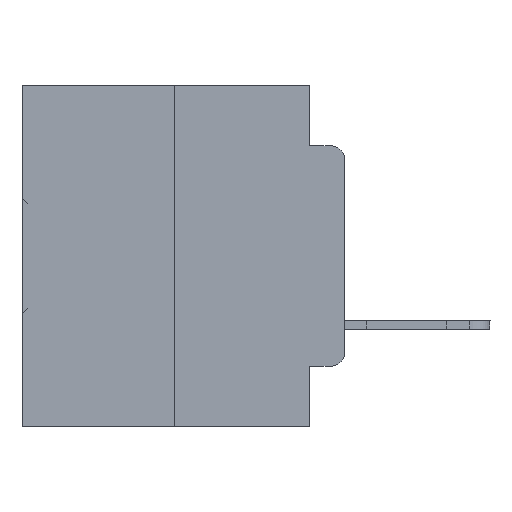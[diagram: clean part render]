
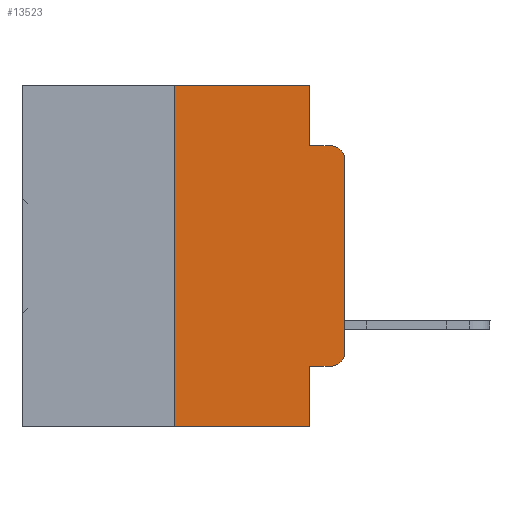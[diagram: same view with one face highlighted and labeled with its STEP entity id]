
A CAD part, left-side view. The second image highlights one B-rep face of the part: STEP entity #13523.
In plain terms, the highlighted planar face has unit normal (-1, 0, 0).
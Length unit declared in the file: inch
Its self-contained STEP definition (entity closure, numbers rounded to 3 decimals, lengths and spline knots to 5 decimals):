
#592 = EDGE_LOOP ( 'NONE', ( #31314, #16976, #10847, #1196, #27279, #27084, #24751, #25529, #22834, #14089 ) ) ;
#767 = CIRCLE ( 'NONE', #9210, 0.02 ) ;
#1196 = ORIENTED_EDGE ( 'NONE', *, *, #12137, .F. ) ;
#1541 = EDGE_CURVE ( 'NONE', #3699, #8849, #767, .T. ) ;
#2777 = DIRECTION ( 'NONE',  ( -1., 0., 0. ) ) ;
#3699 = VERTEX_POINT ( 'NONE', #29137 ) ;
#4284 = VECTOR ( 'NONE', #35732, 39.37008 ) ;
#4747 = CARTESIAN_POINT ( 'NONE',  ( 0., 0.051, -0.0885 ) ) ;
#5040 = DIRECTION ( 'NONE',  ( 0., 0., -1. ) ) ;
#5095 = VERTEX_POINT ( 'NONE', #4747 ) ;
#5227 = CARTESIAN_POINT ( 'NONE',  ( 0., 0.02, -0.3915 ) ) ;
#5934 = CARTESIAN_POINT ( 'NONE',  ( 0., 0.02, -0.1085 ) ) ;
#6182 = DIRECTION ( 'NONE',  ( 0., 0., 1. ) ) ;
#6283 = LINE ( 'NONE', #27998, #31683 ) ;
#6561 = CARTESIAN_POINT ( 'NONE',  ( 0., 0., -0.3915 ) ) ;
#7184 = CARTESIAN_POINT ( 'NONE',  ( 0., 0.25, -0.5 ) ) ;
#7583 = VERTEX_POINT ( 'NONE', #31201 ) ;
#8425 = LINE ( 'NONE', #22892, #10570 ) ;
#8849 = VERTEX_POINT ( 'NONE', #6561 ) ;
#9210 = AXIS2_PLACEMENT_3D ( 'NONE', #5227, #2777, #22008 ) ;
#10047 = VECTOR ( 'NONE', #14059, 39.37008 ) ;
#10087 = DIRECTION ( 'NONE',  ( 0., 0., 1. ) ) ;
#10299 = CARTESIAN_POINT ( 'NONE',  ( 0., 0.051, 0. ) ) ;
#10502 = VERTEX_POINT ( 'NONE', #25774 ) ;
#10570 = VECTOR ( 'NONE', #33578, 39.37008 ) ;
#10847 = ORIENTED_EDGE ( 'NONE', *, *, #14008, .F. ) ;
#11487 = VECTOR ( 'NONE', #10087, 39.37008 ) ;
#11555 = LINE ( 'NONE', #27419, #4284 ) ;
#11594 = EDGE_CURVE ( 'NONE', #13552, #33379, #26052, .T. ) ;
#12137 = EDGE_CURVE ( 'NONE', #33379, #5095, #21808, .T. ) ;
#12580 = CARTESIAN_POINT ( 'NONE',  ( 0., 0.02, -0.0885 ) ) ;
#12822 = CIRCLE ( 'NONE', #16520, 0.02 ) ;
#13139 = VECTOR ( 'NONE', #26308, 39.37008 ) ;
#13523 = ADVANCED_FACE ( 'NONE', ( #30210 ), #13792, .F. ) ;
#13552 = VERTEX_POINT ( 'NONE', #16355 ) ;
#13792 = PLANE ( 'NONE',  #30494 ) ;
#14008 = EDGE_CURVE ( 'NONE', #5095, #34127, #33595, .T. ) ;
#14059 = DIRECTION ( 'NONE',  ( 0., 0., -1. ) ) ;
#14089 = ORIENTED_EDGE ( 'NONE', *, *, #1541, .T. ) ;
#14116 = LINE ( 'NONE', #23769, #11487 ) ;
#15572 = LINE ( 'NONE', #32622, #29811 ) ;
#16113 = EDGE_CURVE ( 'NONE', #19911, #13552, #6283, .T. ) ;
#16129 = DIRECTION ( 'NONE',  ( 0., -1., 0. ) ) ;
#16355 = CARTESIAN_POINT ( 'NONE',  ( 0., 0.25, 0. ) ) ;
#16520 = AXIS2_PLACEMENT_3D ( 'NONE', #5934, #16665, #19462 ) ;
#16665 = DIRECTION ( 'NONE',  ( -1., 0., 0. ) ) ;
#16945 = EDGE_CURVE ( 'NONE', #8849, #10502, #14116, .T. ) ;
#16976 = ORIENTED_EDGE ( 'NONE', *, *, #34427, .T. ) ;
#19174 = CARTESIAN_POINT ( 'NONE',  ( 0., 0.051, -0.0885 ) ) ;
#19295 = DIRECTION ( 'NONE',  ( 0., -1., 0. ) ) ;
#19462 = DIRECTION ( 'NONE',  ( 0., 0., -1. ) ) ;
#19911 = VERTEX_POINT ( 'NONE', #7184 ) ;
#20550 = CARTESIAN_POINT ( 'NONE',  ( 0., 0.473, 0. ) ) ;
#21808 = LINE ( 'NONE', #33330, #10047 ) ;
#22008 = DIRECTION ( 'NONE',  ( 0., 0., -1. ) ) ;
#22834 = ORIENTED_EDGE ( 'NONE', *, *, #29122, .T. ) ;
#22892 = CARTESIAN_POINT ( 'NONE',  ( 0., 0.473, -0.5 ) ) ;
#23769 = CARTESIAN_POINT ( 'NONE',  ( 0., 0., 0. ) ) ;
#24235 = CARTESIAN_POINT ( 'NONE',  ( 0., 0.051, -0.5 ) ) ;
#24435 = DIRECTION ( 'NONE',  ( 1., 0., 0. ) ) ;
#24751 = ORIENTED_EDGE ( 'NONE', *, *, #35591, .T. ) ;
#25529 = ORIENTED_EDGE ( 'NONE', *, *, #29598, .F. ) ;
#25774 = CARTESIAN_POINT ( 'NONE',  ( 0., 0., -0.1085 ) ) ;
#26052 = LINE ( 'NONE', #20550, #13139 ) ;
#26308 = DIRECTION ( 'NONE',  ( 0., -1., 0. ) ) ;
#27084 = ORIENTED_EDGE ( 'NONE', *, *, #16113, .F. ) ;
#27279 = ORIENTED_EDGE ( 'NONE', *, *, #11594, .F. ) ;
#27419 = CARTESIAN_POINT ( 'NONE',  ( 0., 0.051, 0. ) ) ;
#27620 = VECTOR ( 'NONE', #19295, 39.37008 ) ;
#27998 = CARTESIAN_POINT ( 'NONE',  ( 0., 0.25, 0. ) ) ;
#29122 = EDGE_CURVE ( 'NONE', #7583, #3699, #15572, .T. ) ;
#29137 = CARTESIAN_POINT ( 'NONE',  ( 0., 0.02, -0.4115 ) ) ;
#29598 = EDGE_CURVE ( 'NONE', #7583, #35391, #11555, .T. ) ;
#29811 = VECTOR ( 'NONE', #16129, 39.37008 ) ;
#30210 = FACE_OUTER_BOUND ( 'NONE', #592, .T. ) ;
#30494 = AXIS2_PLACEMENT_3D ( 'NONE', #35282, #24435, #5040 ) ;
#31201 = CARTESIAN_POINT ( 'NONE',  ( 0., 0.051, -0.4115 ) ) ;
#31314 = ORIENTED_EDGE ( 'NONE', *, *, #16945, .T. ) ;
#31683 = VECTOR ( 'NONE', #6182, 39.37008 ) ;
#32622 = CARTESIAN_POINT ( 'NONE',  ( 0., 0.051, -0.4115 ) ) ;
#33330 = CARTESIAN_POINT ( 'NONE',  ( 0., 0.051, 0. ) ) ;
#33379 = VERTEX_POINT ( 'NONE', #10299 ) ;
#33578 = DIRECTION ( 'NONE',  ( 0., -1., 0. ) ) ;
#33595 = LINE ( 'NONE', #19174, #27620 ) ;
#34127 = VERTEX_POINT ( 'NONE', #12580 ) ;
#34427 = EDGE_CURVE ( 'NONE', #10502, #34127, #12822, .T. ) ;
#35282 = CARTESIAN_POINT ( 'NONE',  ( 0., 0.473, 0. ) ) ;
#35391 = VERTEX_POINT ( 'NONE', #24235 ) ;
#35591 = EDGE_CURVE ( 'NONE', #19911, #35391, #8425, .T. ) ;
#35732 = DIRECTION ( 'NONE',  ( 0., 0., -1. ) ) ;
